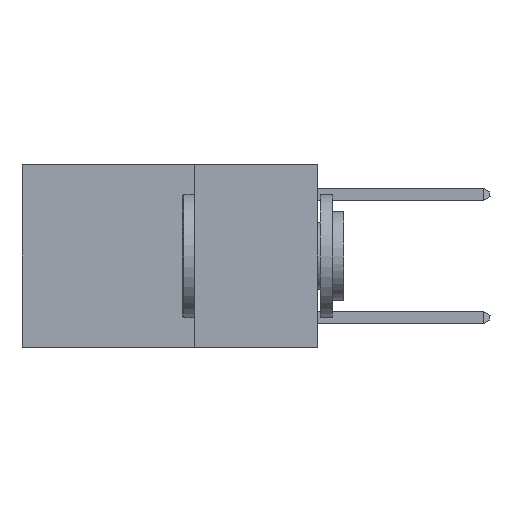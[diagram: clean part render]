
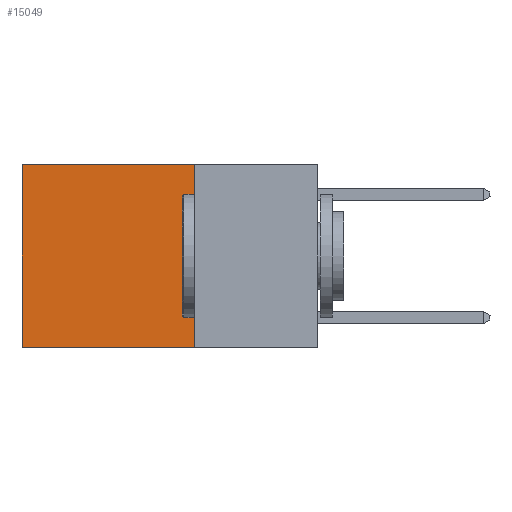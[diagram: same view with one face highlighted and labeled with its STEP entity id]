
A CAD part, left-side view. The second image highlights one B-rep face of the part: STEP entity #15049.
In plain terms, the highlighted planar face has unit normal (-1, 0, 0).
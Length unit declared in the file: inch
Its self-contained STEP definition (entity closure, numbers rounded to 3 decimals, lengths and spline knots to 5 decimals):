
#14 = DIRECTION ( 'NONE',  ( 1., 0., 0. ) ) ;
#288 = EDGE_CURVE ( 'NONE', #1521, #5258, #13549, .T. ) ;
#621 = CARTESIAN_POINT ( 'NONE',  ( 0.2625, 0.25, -0.37 ) ) ;
#997 = ORIENTED_EDGE ( 'NONE', *, *, #6770, .T. ) ;
#1091 = DIRECTION ( 'NONE',  ( 0., 0., -1. ) ) ;
#1134 = ORIENTED_EDGE ( 'NONE', *, *, #13205, .T. ) ;
#1329 = EDGE_CURVE ( 'NONE', #10824, #1521, #6968, .T. ) ;
#1521 = VERTEX_POINT ( 'NONE', #621 ) ;
#3301 = ORIENTED_EDGE ( 'NONE', *, *, #1329, .F. ) ;
#3302 = VERTEX_POINT ( 'NONE', #9380 ) ;
#3910 = DIRECTION ( 'NONE',  ( 0., 1., 0. ) ) ;
#4105 = CARTESIAN_POINT ( 'NONE',  ( 0.2625, 0.6, -0.37 ) ) ;
#4886 = DIRECTION ( 'NONE',  ( 0., 0., -1. ) ) ;
#5258 = VERTEX_POINT ( 'NONE', #4105 ) ;
#5357 = EDGE_LOOP ( 'NONE', ( #997, #6025, #3301, #1134 ) ) ;
#5795 = PLANE ( 'NONE',  #12390 ) ;
#6025 = ORIENTED_EDGE ( 'NONE', *, *, #288, .F. ) ;
#6576 = VECTOR ( 'NONE', #1091, 39.37008 ) ;
#6770 = EDGE_CURVE ( 'NONE', #3302, #5258, #11493, .T. ) ;
#6968 = LINE ( 'NONE', #8176, #8224 ) ;
#7019 = CARTESIAN_POINT ( 'NONE',  ( 0.2625, 0.25, 0. ) ) ;
#7889 = VECTOR ( 'NONE', #14948, 39.37008 ) ;
#8176 = CARTESIAN_POINT ( 'NONE',  ( 0.2625, 0.25, 0. ) ) ;
#8224 = VECTOR ( 'NONE', #4886, 39.37008 ) ;
#8485 = CARTESIAN_POINT ( 'NONE',  ( 0.2625, 0.25, 0. ) ) ;
#9150 = FACE_OUTER_BOUND ( 'NONE', #5357, .T. ) ;
#9380 = CARTESIAN_POINT ( 'NONE',  ( 0.2625, 0.6, 0. ) ) ;
#9553 = LINE ( 'NONE', #8485, #14217 ) ;
#10742 = CARTESIAN_POINT ( 'NONE',  ( 0.2625, 0.25, 0. ) ) ;
#10824 = VERTEX_POINT ( 'NONE', #10742 ) ;
#11493 = LINE ( 'NONE', #14027, #6576 ) ;
#12390 = AXIS2_PLACEMENT_3D ( 'NONE', #7019, #14, #13860 ) ;
#12540 = CARTESIAN_POINT ( 'NONE',  ( 0.2625, 0.25, -0.37 ) ) ;
#13205 = EDGE_CURVE ( 'NONE', #10824, #3302, #9553, .T. ) ;
#13549 = LINE ( 'NONE', #12540, #7889 ) ;
#13860 = DIRECTION ( 'NONE',  ( 0., 0., -1. ) ) ;
#14027 = CARTESIAN_POINT ( 'NONE',  ( 0.2625, 0.6, 0. ) ) ;
#14217 = VECTOR ( 'NONE', #3910, 39.37008 ) ;
#14948 = DIRECTION ( 'NONE',  ( 0., 1., 0. ) ) ;
#15049 = ADVANCED_FACE ( 'NONE', ( #9150 ), #5795, .F. ) ;
